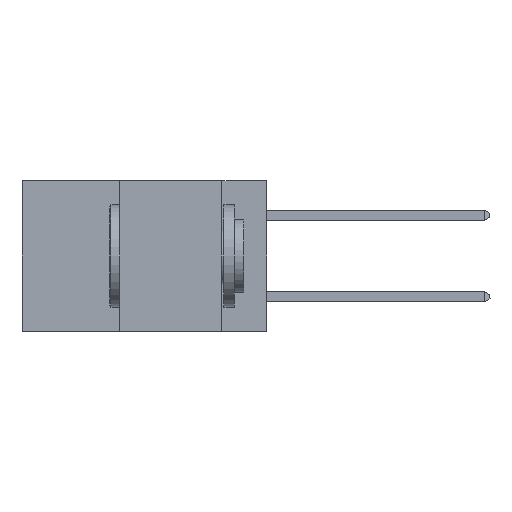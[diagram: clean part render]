
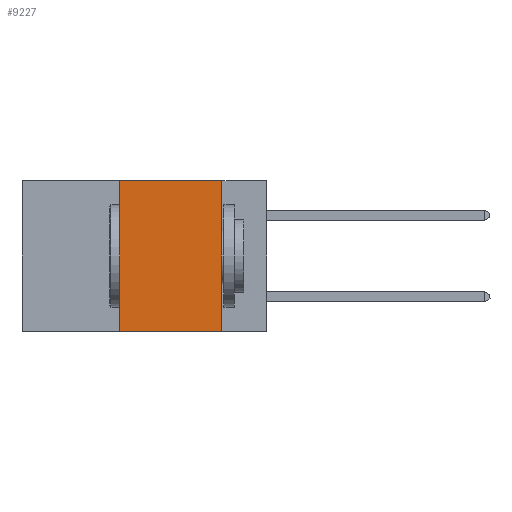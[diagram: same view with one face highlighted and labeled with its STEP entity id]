
A CAD part, left-side view. The second image highlights one B-rep face of the part: STEP entity #9227.
In plain terms, the highlighted planar face has unit normal (-1, 0, 0).
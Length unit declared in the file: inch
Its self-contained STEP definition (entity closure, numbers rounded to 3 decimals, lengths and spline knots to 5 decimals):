
#94 = CARTESIAN_POINT ( 'NONE',  ( 0., 0.36, 0. ) ) ;
#685 = ORIENTED_EDGE ( 'NONE', *, *, #4899, .T. ) ;
#1053 = FACE_OUTER_BOUND ( 'NONE', #8001, .T. ) ;
#1211 = EDGE_CURVE ( 'NONE', #7763, #1502, #4283, .T. ) ;
#1280 = EDGE_CURVE ( 'NONE', #6113, #6545, #6961, .T. ) ;
#1502 = VERTEX_POINT ( 'NONE', #10022 ) ;
#1623 = VECTOR ( 'NONE', #10149, 39.37008 ) ;
#2122 = VECTOR ( 'NONE', #5957, 39.37008 ) ;
#2191 = DIRECTION ( 'NONE',  ( 0., -1., 0. ) ) ;
#2611 = ORIENTED_EDGE ( 'NONE', *, *, #1211, .F. ) ;
#3116 = ORIENTED_EDGE ( 'NONE', *, *, #4810, .F. ) ;
#3149 = DIRECTION ( 'NONE',  ( 0., 0., -1. ) ) ;
#3212 = VECTOR ( 'NONE', #2191, 39.37008 ) ;
#3716 = CARTESIAN_POINT ( 'NONE',  ( 0., 0.36, -0.37 ) ) ;
#4283 = LINE ( 'NONE', #94, #11598 ) ;
#4701 = DIRECTION ( 'NONE',  ( 0., 0., 1. ) ) ;
#4810 = EDGE_CURVE ( 'NONE', #1502, #6113, #10704, .T. ) ;
#4899 = EDGE_CURVE ( 'NONE', #7763, #6545, #11406, .T. ) ;
#5816 = CARTESIAN_POINT ( 'NONE',  ( 0., 0.11, -0.37 ) ) ;
#5881 = CARTESIAN_POINT ( 'NONE',  ( 0., 0.6, 0. ) ) ;
#5957 = DIRECTION ( 'NONE',  ( 0., -1., 0. ) ) ;
#6093 = ORIENTED_EDGE ( 'NONE', *, *, #1280, .F. ) ;
#6113 = VERTEX_POINT ( 'NONE', #8376 ) ;
#6415 = CARTESIAN_POINT ( 'NONE',  ( 0., 0.11, 0. ) ) ;
#6545 = VERTEX_POINT ( 'NONE', #5816 ) ;
#6784 = CARTESIAN_POINT ( 'NONE',  ( 0., 0.6, 0. ) ) ;
#6961 = LINE ( 'NONE', #6415, #1623 ) ;
#7645 = PLANE ( 'NONE',  #7762 ) ;
#7762 = AXIS2_PLACEMENT_3D ( 'NONE', #6784, #8730, #3149 ) ;
#7763 = VERTEX_POINT ( 'NONE', #3716 ) ;
#8001 = EDGE_LOOP ( 'NONE', ( #6093, #3116, #2611, #685 ) ) ;
#8376 = CARTESIAN_POINT ( 'NONE',  ( 0., 0.11, 0. ) ) ;
#8730 = DIRECTION ( 'NONE',  ( 1., 0., 0. ) ) ;
#9227 = ADVANCED_FACE ( 'NONE', ( #1053 ), #7645, .F. ) ;
#10022 = CARTESIAN_POINT ( 'NONE',  ( 0., 0.36, 0. ) ) ;
#10149 = DIRECTION ( 'NONE',  ( 0., 0., -1. ) ) ;
#10704 = LINE ( 'NONE', #5881, #3212 ) ;
#11397 = CARTESIAN_POINT ( 'NONE',  ( 0., 0.6, -0.37 ) ) ;
#11406 = LINE ( 'NONE', #11397, #2122 ) ;
#11598 = VECTOR ( 'NONE', #4701, 39.37008 ) ;
